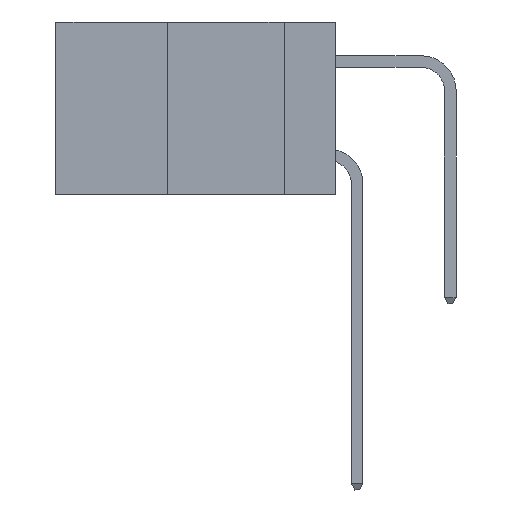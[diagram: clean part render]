
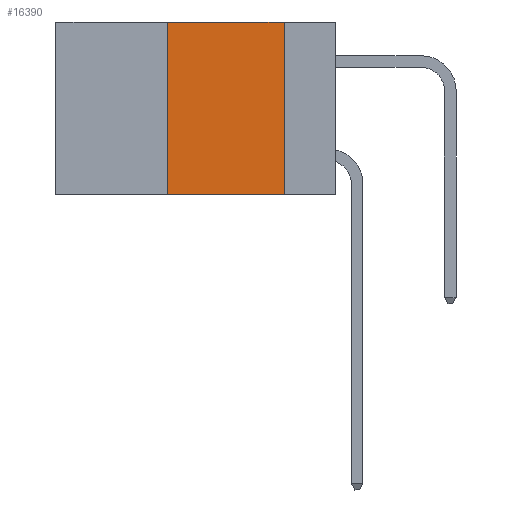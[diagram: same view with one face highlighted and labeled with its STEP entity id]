
A CAD part, left-side view. The second image highlights one B-rep face of the part: STEP entity #16390.
In plain terms, the highlighted planar face has unit normal (-1, 0, 0).
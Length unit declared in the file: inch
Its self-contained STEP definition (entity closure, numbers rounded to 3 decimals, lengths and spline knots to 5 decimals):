
#8 = CARTESIAN_POINT ( 'NONE',  ( 0., 0.36, -0.37 ) ) ;
#149 = LINE ( 'NONE', #11813, #10193 ) ;
#469 = PLANE ( 'NONE',  #1421 ) ;
#549 = CARTESIAN_POINT ( 'NONE',  ( 0., 0.11, 0. ) ) ;
#597 = DIRECTION ( 'NONE',  ( 0., 0., -1. ) ) ;
#1062 = CARTESIAN_POINT ( 'NONE',  ( 0., 0.6, 0. ) ) ;
#1421 = AXIS2_PLACEMENT_3D ( 'NONE', #1827, #11343, #3331 ) ;
#1827 = CARTESIAN_POINT ( 'NONE',  ( 0., 0.6, 0. ) ) ;
#3331 = DIRECTION ( 'NONE',  ( 0., 0., -1. ) ) ;
#3901 = EDGE_CURVE ( 'NONE', #15503, #12022, #149, .T. ) ;
#4595 = EDGE_CURVE ( 'NONE', #14399, #12022, #4874, .T. ) ;
#4874 = LINE ( 'NONE', #549, #8043 ) ;
#4910 = VECTOR ( 'NONE', #11844, 39.37008 ) ;
#6286 = LINE ( 'NONE', #16536, #9413 ) ;
#7009 = EDGE_LOOP ( 'NONE', ( #13416, #12738, #10689, #9431 ) ) ;
#8043 = VECTOR ( 'NONE', #597, 39.37008 ) ;
#8320 = CARTESIAN_POINT ( 'NONE',  ( 0., 0.11, 0. ) ) ;
#9413 = VECTOR ( 'NONE', #12741, 39.37008 ) ;
#9431 = ORIENTED_EDGE ( 'NONE', *, *, #3901, .T. ) ;
#10193 = VECTOR ( 'NONE', #16837, 39.37008 ) ;
#10514 = VERTEX_POINT ( 'NONE', #15007 ) ;
#10689 = ORIENTED_EDGE ( 'NONE', *, *, #16814, .F. ) ;
#10831 = EDGE_CURVE ( 'NONE', #10514, #14399, #15737, .T. ) ;
#11343 = DIRECTION ( 'NONE',  ( 1., 0., 0. ) ) ;
#11813 = CARTESIAN_POINT ( 'NONE',  ( 0., 0.6, -0.37 ) ) ;
#11844 = DIRECTION ( 'NONE',  ( 0., -1., 0. ) ) ;
#12022 = VERTEX_POINT ( 'NONE', #13799 ) ;
#12738 = ORIENTED_EDGE ( 'NONE', *, *, #10831, .F. ) ;
#12741 = DIRECTION ( 'NONE',  ( 0., 0., 1. ) ) ;
#13416 = ORIENTED_EDGE ( 'NONE', *, *, #4595, .F. ) ;
#13799 = CARTESIAN_POINT ( 'NONE',  ( 0., 0.11, -0.37 ) ) ;
#14399 = VERTEX_POINT ( 'NONE', #8320 ) ;
#15007 = CARTESIAN_POINT ( 'NONE',  ( 0., 0.36, 0. ) ) ;
#15503 = VERTEX_POINT ( 'NONE', #8 ) ;
#15737 = LINE ( 'NONE', #1062, #4910 ) ;
#16390 = ADVANCED_FACE ( 'NONE', ( #16550 ), #469, .F. ) ;
#16536 = CARTESIAN_POINT ( 'NONE',  ( 0., 0.36, 0. ) ) ;
#16550 = FACE_OUTER_BOUND ( 'NONE', #7009, .T. ) ;
#16814 = EDGE_CURVE ( 'NONE', #15503, #10514, #6286, .T. ) ;
#16837 = DIRECTION ( 'NONE',  ( 0., -1., 0. ) ) ;
